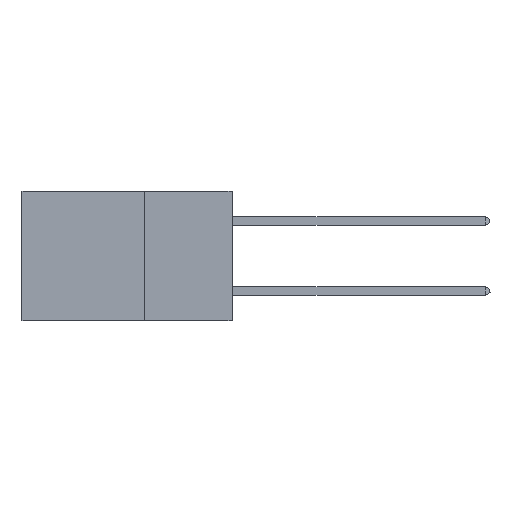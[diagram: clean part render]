
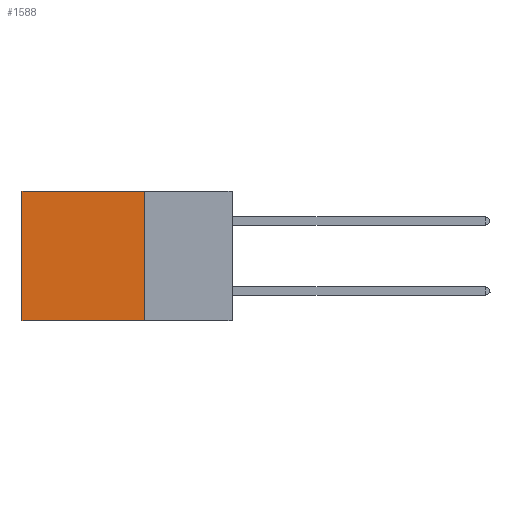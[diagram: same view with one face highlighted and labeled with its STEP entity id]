
A CAD part, left-side view. The second image highlights one B-rep face of the part: STEP entity #1588.
In plain terms, the highlighted planar face has unit normal (-1, 0, 0).
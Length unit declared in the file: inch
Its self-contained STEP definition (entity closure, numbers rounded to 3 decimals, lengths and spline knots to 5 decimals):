
#180 = PLANE ( 'NONE',  #199 ) ;
#199 = AXIS2_PLACEMENT_3D ( 'NONE', #19836, #267, #12743 ) ;
#267 = DIRECTION ( 'NONE',  ( 1., 0., 0. ) ) ;
#439 = CARTESIAN_POINT ( 'NONE',  ( 0.2875, 0.25, 0. ) ) ;
#1556 = LINE ( 'NONE', #18856, #9907 ) ;
#1588 = ADVANCED_FACE ( 'NONE', ( #19442 ), #180, .F. ) ;
#1633 = EDGE_CURVE ( 'NONE', #5616, #13059, #14663, .T. ) ;
#3637 = DIRECTION ( 'NONE',  ( 0., 0., -1. ) ) ;
#3777 = VERTEX_POINT ( 'NONE', #3985 ) ;
#3820 = VECTOR ( 'NONE', #20890, 39.37008 ) ;
#3856 = LINE ( 'NONE', #17581, #11924 ) ;
#3985 = CARTESIAN_POINT ( 'NONE',  ( 0.2875, 0.6, -0.37 ) ) ;
#4421 = EDGE_LOOP ( 'NONE', ( #10244, #8140, #11719, #21315 ) ) ;
#5616 = VERTEX_POINT ( 'NONE', #439 ) ;
#7420 = VERTEX_POINT ( 'NONE', #9858 ) ;
#7774 = LINE ( 'NONE', #16294, #19781 ) ;
#8140 = ORIENTED_EDGE ( 'NONE', *, *, #19530, .F. ) ;
#9858 = CARTESIAN_POINT ( 'NONE',  ( 0.2875, 0.6, 0. ) ) ;
#9907 = VECTOR ( 'NONE', #19170, 39.37008 ) ;
#10244 = ORIENTED_EDGE ( 'NONE', *, *, #15519, .T. ) ;
#11719 = ORIENTED_EDGE ( 'NONE', *, *, #1633, .F. ) ;
#11924 = VECTOR ( 'NONE', #3637, 39.37008 ) ;
#12743 = DIRECTION ( 'NONE',  ( 0., 0., -1. ) ) ;
#13059 = VERTEX_POINT ( 'NONE', #22894 ) ;
#14312 = EDGE_CURVE ( 'NONE', #5616, #7420, #1556, .T. ) ;
#14663 = LINE ( 'NONE', #22607, #3820 ) ;
#15519 = EDGE_CURVE ( 'NONE', #7420, #3777, #3856, .T. ) ;
#16294 = CARTESIAN_POINT ( 'NONE',  ( 0.2875, 0.25, -0.37 ) ) ;
#17581 = CARTESIAN_POINT ( 'NONE',  ( 0.2875, 0.6, 0. ) ) ;
#18077 = DIRECTION ( 'NONE',  ( 0., 1., 0. ) ) ;
#18856 = CARTESIAN_POINT ( 'NONE',  ( 0.2875, 0.25, 0. ) ) ;
#19170 = DIRECTION ( 'NONE',  ( 0., 1., 0. ) ) ;
#19442 = FACE_OUTER_BOUND ( 'NONE', #4421, .T. ) ;
#19530 = EDGE_CURVE ( 'NONE', #13059, #3777, #7774, .T. ) ;
#19781 = VECTOR ( 'NONE', #18077, 39.37008 ) ;
#19836 = CARTESIAN_POINT ( 'NONE',  ( 0.2875, 0.25, 0. ) ) ;
#20890 = DIRECTION ( 'NONE',  ( 0., 0., -1. ) ) ;
#21315 = ORIENTED_EDGE ( 'NONE', *, *, #14312, .T. ) ;
#22607 = CARTESIAN_POINT ( 'NONE',  ( 0.2875, 0.25, 0. ) ) ;
#22894 = CARTESIAN_POINT ( 'NONE',  ( 0.2875, 0.25, -0.37 ) ) ;
